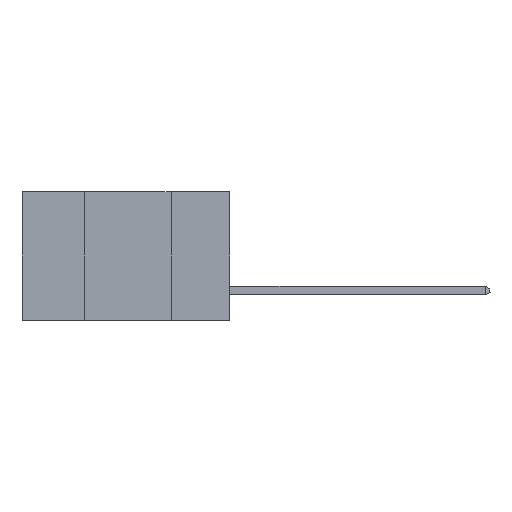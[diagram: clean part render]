
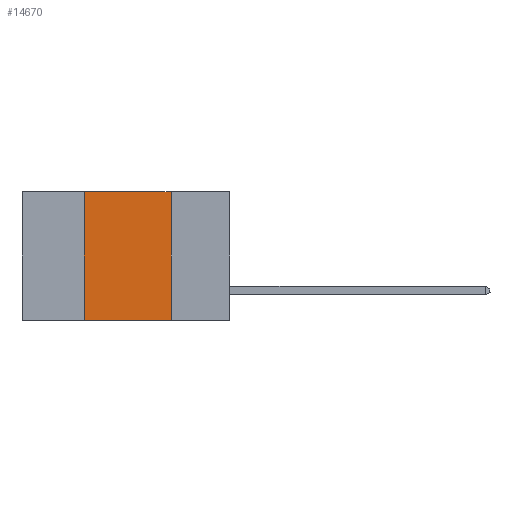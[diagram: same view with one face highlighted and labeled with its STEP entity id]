
A CAD part, left-side view. The second image highlights one B-rep face of the part: STEP entity #14670.
In plain terms, the highlighted planar face has unit normal (-1, 0, 0).
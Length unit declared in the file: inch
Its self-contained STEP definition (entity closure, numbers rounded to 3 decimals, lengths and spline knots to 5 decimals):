
#56 = ORIENTED_EDGE ( 'NONE', *, *, #8137, .F. ) ;
#215 = CARTESIAN_POINT ( 'NONE',  ( 0., 0.42, 0. ) ) ;
#626 = DIRECTION ( 'NONE',  ( 0., 0., -1. ) ) ;
#634 = CARTESIAN_POINT ( 'NONE',  ( 0., 0.17, 0. ) ) ;
#1102 = DIRECTION ( 'NONE',  ( 0., -1., 0. ) ) ;
#1129 = AXIS2_PLACEMENT_3D ( 'NONE', #2160, #15108, #626 ) ;
#2160 = CARTESIAN_POINT ( 'NONE',  ( 0., 0.6, 0. ) ) ;
#2690 = LINE ( 'NONE', #215, #13634 ) ;
#4456 = VERTEX_POINT ( 'NONE', #16845 ) ;
#5096 = DIRECTION ( 'NONE',  ( 0., 0., 1. ) ) ;
#6646 = LINE ( 'NONE', #9003, #15398 ) ;
#7439 = LINE ( 'NONE', #12742, #19760 ) ;
#7617 = ORIENTED_EDGE ( 'NONE', *, *, #13951, .F. ) ;
#7967 = DIRECTION ( 'NONE',  ( 0., -1., 0. ) ) ;
#8137 = EDGE_CURVE ( 'NONE', #19544, #4456, #15140, .T. ) ;
#8315 = ORIENTED_EDGE ( 'NONE', *, *, #20467, .T. ) ;
#9003 = CARTESIAN_POINT ( 'NONE',  ( 0., 0.6, 0. ) ) ;
#9828 = CARTESIAN_POINT ( 'NONE',  ( 0., 0.17, 0. ) ) ;
#10075 = PLANE ( 'NONE',  #1129 ) ;
#10127 = VECTOR ( 'NONE', #18372, 39.37008 ) ;
#10717 = EDGE_LOOP ( 'NONE', ( #56, #7617, #18809, #8315 ) ) ;
#10822 = FACE_OUTER_BOUND ( 'NONE', #10717, .T. ) ;
#12111 = CARTESIAN_POINT ( 'NONE',  ( 0., 0.42, -0.37 ) ) ;
#12742 = CARTESIAN_POINT ( 'NONE',  ( 0., 0.6, -0.37 ) ) ;
#13634 = VECTOR ( 'NONE', #5096, 39.37008 ) ;
#13951 = EDGE_CURVE ( 'NONE', #19989, #19544, #6646, .T. ) ;
#14670 = ADVANCED_FACE ( 'NONE', ( #10822 ), #10075, .F. ) ;
#15108 = DIRECTION ( 'NONE',  ( 1., 0., 0. ) ) ;
#15140 = LINE ( 'NONE', #634, #10127 ) ;
#15398 = VECTOR ( 'NONE', #1102, 39.37008 ) ;
#15687 = CARTESIAN_POINT ( 'NONE',  ( 0., 0.42, 0. ) ) ;
#16845 = CARTESIAN_POINT ( 'NONE',  ( 0., 0.17, -0.37 ) ) ;
#18372 = DIRECTION ( 'NONE',  ( 0., 0., -1. ) ) ;
#18430 = EDGE_CURVE ( 'NONE', #19357, #19989, #2690, .T. ) ;
#18809 = ORIENTED_EDGE ( 'NONE', *, *, #18430, .F. ) ;
#19357 = VERTEX_POINT ( 'NONE', #12111 ) ;
#19544 = VERTEX_POINT ( 'NONE', #9828 ) ;
#19760 = VECTOR ( 'NONE', #7967, 39.37008 ) ;
#19989 = VERTEX_POINT ( 'NONE', #15687 ) ;
#20467 = EDGE_CURVE ( 'NONE', #19357, #4456, #7439, .T. ) ;
